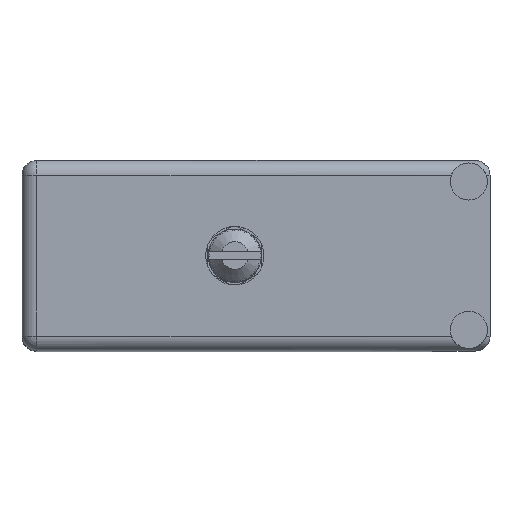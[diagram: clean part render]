
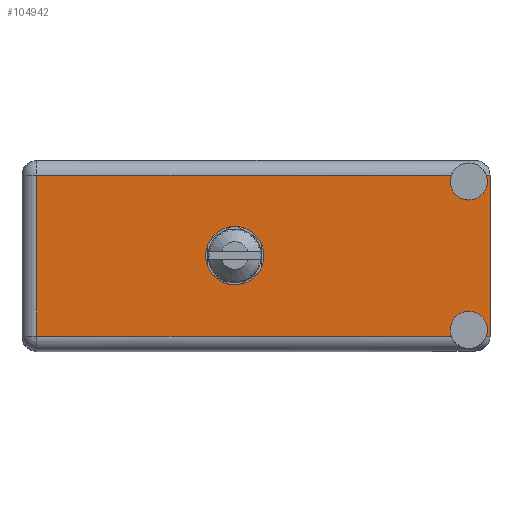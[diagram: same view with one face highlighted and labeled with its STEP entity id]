
A CAD part, top view. The second image highlights one B-rep face of the part: STEP entity #104942.
In plain terms, the highlighted face is planar.
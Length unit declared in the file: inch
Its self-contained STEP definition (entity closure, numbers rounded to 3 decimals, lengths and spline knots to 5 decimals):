
#406 = DIRECTION ( 'NONE',  ( -1., 0., 0. ) ) ;
#960 = LINE ( 'NONE', #93615, #25689 ) ;
#1198 = AXIS2_PLACEMENT_3D ( 'NONE', #65898, #7478, #84094 ) ;
#3084 = ORIENTED_EDGE ( 'NONE', *, *, #38523, .F. ) ;
#4586 = DIRECTION ( 'NONE',  ( 0., 1., 0. ) ) ;
#5284 = EDGE_LOOP ( 'NONE', ( #76938, #70429 ) ) ;
#6237 = DIRECTION ( 'NONE',  ( -1., 0., 0. ) ) ;
#7478 = DIRECTION ( 'NONE',  ( 0., 1., 0. ) ) ;
#7800 = CIRCLE ( 'NONE', #14780, 0.1375 ) ;
#7978 = VERTEX_POINT ( 'NONE', #105470 ) ;
#8022 = FACE_BOUND ( 'NONE', #5284, .T. ) ;
#8120 = DIRECTION ( 'NONE',  ( 0., 1., 0. ) ) ;
#11749 = DIRECTION ( 'NONE',  ( 0., 1., 0. ) ) ;
#12018 = DIRECTION ( 'NONE',  ( 0., 1., 0. ) ) ;
#12672 = ORIENTED_EDGE ( 'NONE', *, *, #26514, .T. ) ;
#13727 = DIRECTION ( 'NONE',  ( 0., 0., 1. ) ) ;
#14071 = EDGE_CURVE ( 'NONE', #95520, #60839, #960, .T. ) ;
#14780 = AXIS2_PLACEMENT_3D ( 'NONE', #40091, #8120, #106837 ) ;
#14984 = EDGE_CURVE ( 'NONE', #91884, #95520, #31057, .T. ) ;
#15839 = ORIENTED_EDGE ( 'NONE', *, *, #108915, .F. ) ;
#16108 = VECTOR ( 'NONE', #406, 39.37008 ) ;
#18699 = VERTEX_POINT ( 'NONE', #25463 ) ;
#19154 = ORIENTED_EDGE ( 'NONE', *, *, #92203, .F. ) ;
#22378 = ORIENTED_EDGE ( 'NONE', *, *, #14984, .T. ) ;
#25463 = CARTESIAN_POINT ( 'NONE',  ( 2.108, 1.566, -0.187 ) ) ;
#25689 = VECTOR ( 'NONE', #45062, 39.37008 ) ;
#26514 = EDGE_CURVE ( 'NONE', #54718, #78627, #109086, .T. ) ;
#28253 = CARTESIAN_POINT ( 'NONE',  ( 2.108, 1.566, -0.0995 ) ) ;
#29015 = CARTESIAN_POINT ( 'NONE',  ( 2.208, 1.566, -0.07 ) ) ;
#30072 = DIRECTION ( 'NONE',  ( 1., 0., 0. ) ) ;
#30492 = VERTEX_POINT ( 'NONE', #87401 ) ;
#31057 = LINE ( 'NONE', #90628, #81824 ) ;
#36355 = CARTESIAN_POINT ( 'NONE',  ( 1.004, 1.566, -0.312 ) ) ;
#36377 = ORIENTED_EDGE ( 'NONE', *, *, #48845, .T. ) ;
#36938 = ORIENTED_EDGE ( 'NONE', *, *, #56801, .T. ) ;
#37985 = LINE ( 'NONE', #38516, #55289 ) ;
#38516 = CARTESIAN_POINT ( 'NONE',  ( 2.208, 1.566, 0. ) ) ;
#38523 = EDGE_CURVE ( 'NONE', #54681, #18699, #63790, .T. ) ;
#40091 = CARTESIAN_POINT ( 'NONE',  ( 1.004, 1.566, -0.4495 ) ) ;
#41448 = AXIS2_PLACEMENT_3D ( 'NONE', #108944, #59814, #93466 ) ;
#42480 = CARTESIAN_POINT ( 'NONE',  ( 2.108, 1.566, -0.7995 ) ) ;
#45062 = DIRECTION ( 'NONE',  ( 0., 0., 1. ) ) ;
#48845 = EDGE_CURVE ( 'NONE', #54681, #71021, #61553, .T. ) ;
#49610 = EDGE_CURVE ( 'NONE', #91884, #7978, #57833, .T. ) ;
#51984 = VERTEX_POINT ( 'NONE', #101295 ) ;
#54681 = VERTEX_POINT ( 'NONE', #88755 ) ;
#54718 = VERTEX_POINT ( 'NONE', #84832 ) ;
#55289 = VECTOR ( 'NONE', #13727, 39.37008 ) ;
#56801 = EDGE_CURVE ( 'NONE', #60839, #51984, #85836, .T. ) ;
#57553 = CIRCLE ( 'NONE', #1198, 0.0875 ) ;
#57833 = CIRCLE ( 'NONE', #101862, 0.0875 ) ;
#58469 = ORIENTED_EDGE ( 'NONE', *, *, #75492, .F. ) ;
#58577 = CARTESIAN_POINT ( 'NONE',  ( 0.07, 1.566, -0.829 ) ) ;
#59814 = DIRECTION ( 'NONE',  ( 0., 1., 0. ) ) ;
#60137 = CARTESIAN_POINT ( 'NONE',  ( 2.208, 1.566, -0.07 ) ) ;
#60839 = VERTEX_POINT ( 'NONE', #78913 ) ;
#61553 = LINE ( 'NONE', #29015, #103587 ) ;
#63790 = CIRCLE ( 'NONE', #91767, 0.0875 ) ;
#65898 = CARTESIAN_POINT ( 'NONE',  ( 2.108, 1.566, -0.7995 ) ) ;
#67528 = PLANE ( 'NONE',  #41448 ) ;
#69597 = DIRECTION ( 'NONE',  ( 0., 0., 1. ) ) ;
#69821 = CIRCLE ( 'NONE', #98016, 0.1375 ) ;
#70429 = ORIENTED_EDGE ( 'NONE', *, *, #71539, .F. ) ;
#71021 = VERTEX_POINT ( 'NONE', #60137 ) ;
#71368 = CIRCLE ( 'NONE', #90753, 0.0875 ) ;
#71539 = EDGE_CURVE ( 'NONE', #30492, #86312, #7800, .T. ) ;
#71753 = ORIENTED_EDGE ( 'NONE', *, *, #14071, .T. ) ;
#72439 = EDGE_LOOP ( 'NONE', ( #36938, #58469, #3084, #36377, #19154, #12672, #15839, #80150, #22378, #71753 ) ) ;
#75011 = DIRECTION ( 'NONE',  ( 0., 1., 0. ) ) ;
#75492 = EDGE_CURVE ( 'NONE', #18699, #51984, #71368, .T. ) ;
#75546 = DIRECTION ( 'NONE',  ( 0., 0., 1. ) ) ;
#75955 = CARTESIAN_POINT ( 'NONE',  ( 0., 1.566, -0.829 ) ) ;
#76938 = ORIENTED_EDGE ( 'NONE', *, *, #108313, .F. ) ;
#77548 = DIRECTION ( 'NONE',  ( 1., 0., 0. ) ) ;
#78078 = CARTESIAN_POINT ( 'NONE',  ( 2.19038, 1.566, -0.829 ) ) ;
#78627 = VERTEX_POINT ( 'NONE', #78078 ) ;
#78913 = CARTESIAN_POINT ( 'NONE',  ( 0.07, 1.566, -0.07 ) ) ;
#80150 = ORIENTED_EDGE ( 'NONE', *, *, #49610, .F. ) ;
#81824 = VECTOR ( 'NONE', #6237, 39.37008 ) ;
#84094 = DIRECTION ( 'NONE',  ( 0., 0., 1. ) ) ;
#84162 = CARTESIAN_POINT ( 'NONE',  ( 2.02562, 1.566, -0.829 ) ) ;
#84752 = CARTESIAN_POINT ( 'NONE',  ( 2.208, 1.566, -0.07 ) ) ;
#84756 = DIRECTION ( 'NONE',  ( 0., 0., 1. ) ) ;
#84832 = CARTESIAN_POINT ( 'NONE',  ( 2.208, 1.566, -0.829 ) ) ;
#85836 = LINE ( 'NONE', #84752, #92581 ) ;
#86312 = VERTEX_POINT ( 'NONE', #36355 ) ;
#87401 = CARTESIAN_POINT ( 'NONE',  ( 1.004, 1.566, -0.587 ) ) ;
#88755 = CARTESIAN_POINT ( 'NONE',  ( 2.19038, 1.566, -0.07 ) ) ;
#90628 = CARTESIAN_POINT ( 'NONE',  ( 0., 1.566, -0.829 ) ) ;
#90753 = AXIS2_PLACEMENT_3D ( 'NONE', #95800, #12018, #104640 ) ;
#91767 = AXIS2_PLACEMENT_3D ( 'NONE', #28253, #11749, #69597 ) ;
#91884 = VERTEX_POINT ( 'NONE', #84162 ) ;
#92203 = EDGE_CURVE ( 'NONE', #54718, #71021, #37985, .T. ) ;
#92581 = VECTOR ( 'NONE', #77548, 39.37008 ) ;
#92924 = FACE_OUTER_BOUND ( 'NONE', #72439, .T. ) ;
#93466 = DIRECTION ( 'NONE',  ( 0., 0., 1. ) ) ;
#93583 = CARTESIAN_POINT ( 'NONE',  ( 1.004, 1.566, -0.4495 ) ) ;
#93615 = CARTESIAN_POINT ( 'NONE',  ( 0.07, 1.566, -0.899 ) ) ;
#95520 = VERTEX_POINT ( 'NONE', #58577 ) ;
#95800 = CARTESIAN_POINT ( 'NONE',  ( 2.108, 1.566, -0.0995 ) ) ;
#98016 = AXIS2_PLACEMENT_3D ( 'NONE', #93583, #4586, #84756 ) ;
#101295 = CARTESIAN_POINT ( 'NONE',  ( 2.02562, 1.566, -0.07 ) ) ;
#101862 = AXIS2_PLACEMENT_3D ( 'NONE', #42480, #75011, #75546 ) ;
#103587 = VECTOR ( 'NONE', #30072, 39.37008 ) ;
#104640 = DIRECTION ( 'NONE',  ( 0., 0., 1. ) ) ;
#104942 = ADVANCED_FACE ( 'NONE', ( #8022, #92924 ), #67528, .T. ) ;
#105470 = CARTESIAN_POINT ( 'NONE',  ( 2.108, 1.566, -0.712 ) ) ;
#106837 = DIRECTION ( 'NONE',  ( 0., 0., 1. ) ) ;
#108313 = EDGE_CURVE ( 'NONE', #86312, #30492, #69821, .T. ) ;
#108915 = EDGE_CURVE ( 'NONE', #7978, #78627, #57553, .T. ) ;
#108944 = CARTESIAN_POINT ( 'NONE',  ( 0., 1.566, -0.899 ) ) ;
#109086 = LINE ( 'NONE', #75955, #16108 ) ;
